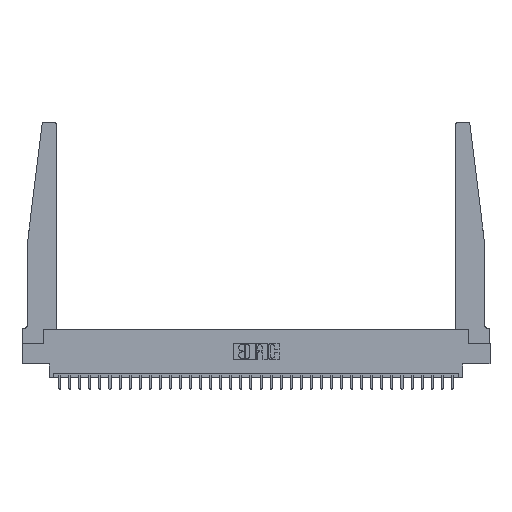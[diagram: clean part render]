
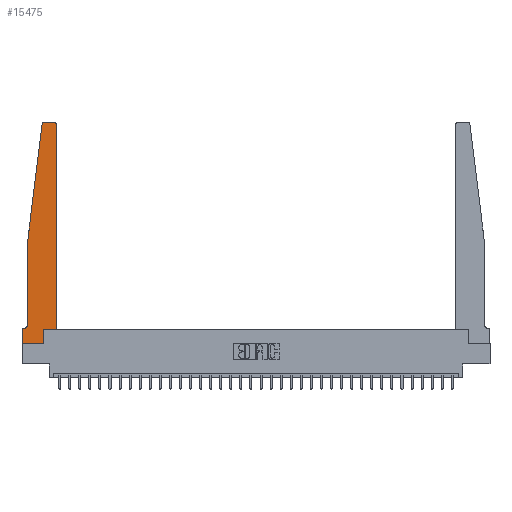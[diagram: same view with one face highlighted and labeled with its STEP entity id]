
A CAD part, top view. The second image highlights one B-rep face of the part: STEP entity #15475.
In plain terms, the highlighted planar face has unit normal (0, 0, 1).
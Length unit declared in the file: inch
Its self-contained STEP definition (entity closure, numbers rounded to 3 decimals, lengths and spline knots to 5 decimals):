
#81 = CARTESIAN_POINT ( 'NONE',  ( 0.395, 2.75, 0.37 ) ) ;
#188 = EDGE_CURVE ( 'NONE', #4004, #19025, #22978, .T. ) ;
#197 = ORIENTED_EDGE ( 'NONE', *, *, #20893, .T. ) ;
#679 = DIRECTION ( 'NONE',  ( 0., -1., 0. ) ) ;
#1126 = CARTESIAN_POINT ( 'NONE',  ( 0.425, 0.18, 0.37 ) ) ;
#2645 = CARTESIAN_POINT ( 'NONE',  ( 0.395, 2.72, 0.37 ) ) ;
#3099 = CARTESIAN_POINT ( 'NONE',  ( 0.065, 1.25, 0.37 ) ) ;
#3260 = CARTESIAN_POINT ( 'NONE',  ( 0.065, 1.25, 0.37 ) ) ;
#3842 = ORIENTED_EDGE ( 'NONE', *, *, #188, .T. ) ;
#3974 = DIRECTION ( 'NONE',  ( 1., 0., 0. ) ) ;
#4004 = VERTEX_POINT ( 'NONE', #18181 ) ;
#4383 = VERTEX_POINT ( 'NONE', #7712 ) ;
#4920 = VECTOR ( 'NONE', #15862, 39.37008 ) ;
#5093 = CARTESIAN_POINT ( 'NONE',  ( 0., 0., 0.37 ) ) ;
#5381 = ORIENTED_EDGE ( 'NONE', *, *, #17141, .T. ) ;
#5448 = VECTOR ( 'NONE', #679, 39.37008 ) ;
#6052 = EDGE_CURVE ( 'NONE', #19632, #29358, #28255, .T. ) ;
#6224 = EDGE_CURVE ( 'NONE', #10576, #30349, #29089, .T. ) ;
#6478 = VECTOR ( 'NONE', #3974, 39.37008 ) ;
#6811 = VERTEX_POINT ( 'NONE', #24458 ) ;
#6896 = CARTESIAN_POINT ( 'NONE',  ( 0.27653, 2.75, 0.37 ) ) ;
#7682 = DIRECTION ( 'NONE',  ( 1., 0., 0. ) ) ;
#7712 = CARTESIAN_POINT ( 'NONE',  ( 0.065, 1.25, 0.37 ) ) ;
#8177 = CARTESIAN_POINT ( 'NONE',  ( 0.2605, 0.18, 0.37 ) ) ;
#8314 = CARTESIAN_POINT ( 'NONE',  ( 0.25, 2.75, 0.37 ) ) ;
#8515 = DIRECTION ( 'NONE',  ( 0., -1., 0. ) ) ;
#9264 = CARTESIAN_POINT ( 'NONE',  ( 0., 0., 0.37 ) ) ;
#9479 = ORIENTED_EDGE ( 'NONE', *, *, #21279, .T. ) ;
#9689 = DIRECTION ( 'NONE',  ( 0., 0., 1. ) ) ;
#9752 = ORIENTED_EDGE ( 'NONE', *, *, #24899, .T. ) ;
#9802 = VECTOR ( 'NONE', #8515, 39.37008 ) ;
#10396 = ORIENTED_EDGE ( 'NONE', *, *, #6224, .T. ) ;
#10576 = VERTEX_POINT ( 'NONE', #6896 ) ;
#10902 = EDGE_CURVE ( 'NONE', #19761, #19632, #23251, .T. ) ;
#11032 = ORIENTED_EDGE ( 'NONE', *, *, #10902, .T. ) ;
#11674 = ORIENTED_EDGE ( 'NONE', *, *, #31141, .T. ) ;
#11796 = VECTOR ( 'NONE', #20056, 39.37008 ) ;
#12055 = CARTESIAN_POINT ( 'NONE',  ( 0.425, 0.18, 0.37 ) ) ;
#12337 = EDGE_CURVE ( 'NONE', #4383, #18650, #25102, .T. ) ;
#12482 = FACE_OUTER_BOUND ( 'NONE', #17894, .T. ) ;
#12603 = VECTOR ( 'NONE', #29712, 39.37008 ) ;
#12979 = CARTESIAN_POINT ( 'NONE',  ( 0.065, 0.1875, 0.37 ) ) ;
#14543 = LINE ( 'NONE', #5093, #21411 ) ;
#14899 = PLANE ( 'NONE',  #20337 ) ;
#15475 = ADVANCED_FACE ( 'NONE', ( #12482 ), #14899, .T. ) ;
#15824 = AXIS2_PLACEMENT_3D ( 'NONE', #2645, #9689, #31714 ) ;
#15862 = DIRECTION ( 'NONE',  ( 0., 1., 0. ) ) ;
#16350 = ORIENTED_EDGE ( 'NONE', *, *, #20463, .T. ) ;
#16833 = VECTOR ( 'NONE', #25554, 39.37008 ) ;
#17141 = EDGE_CURVE ( 'NONE', #29358, #25570, #25386, .T. ) ;
#17362 = CIRCLE ( 'NONE', #15824, 0.03 ) ;
#17663 = CARTESIAN_POINT ( 'NONE',  ( 0.2605, 0.18, 0.37 ) ) ;
#17666 = CARTESIAN_POINT ( 'NONE',  ( 0., 0., 0.37 ) ) ;
#17828 = CARTESIAN_POINT ( 'NONE',  ( 0.2605, 0., 0.37 ) ) ;
#17894 = EDGE_LOOP ( 'NONE', ( #9752, #10396, #197, #23150, #28321, #11674, #3842, #16350, #11032, #21083, #5381, #9479 ) ) ;
#18181 = CARTESIAN_POINT ( 'NONE',  ( 0., 0.1875, 0.37 ) ) ;
#18323 = DIRECTION ( 'NONE',  ( -0.122, -0.992, 0. ) ) ;
#18650 = VERTEX_POINT ( 'NONE', #29242 ) ;
#19025 = VERTEX_POINT ( 'NONE', #9264 ) ;
#19557 = CARTESIAN_POINT ( 'NONE',  ( 0., 0.1875, 0.37 ) ) ;
#19632 = VERTEX_POINT ( 'NONE', #17663 ) ;
#19761 = VERTEX_POINT ( 'NONE', #17828 ) ;
#19867 = LINE ( 'NONE', #8314, #12603 ) ;
#20056 = DIRECTION ( 'NONE',  ( -1., 0., 0. ) ) ;
#20337 = AXIS2_PLACEMENT_3D ( 'NONE', #19557, #29387, #7682 ) ;
#20463 = EDGE_CURVE ( 'NONE', #19025, #19761, #14543, .T. ) ;
#20893 = EDGE_CURVE ( 'NONE', #30349, #4383, #25420, .T. ) ;
#21083 = ORIENTED_EDGE ( 'NONE', *, *, #6052, .T. ) ;
#21279 = EDGE_CURVE ( 'NONE', #25570, #23945, #17362, .T. ) ;
#21411 = VECTOR ( 'NONE', #21940, 39.37008 ) ;
#21899 = CIRCLE ( 'NONE', #26031, 0.05 ) ;
#21940 = DIRECTION ( 'NONE',  ( 1., 0., 0. ) ) ;
#22890 = AXIS2_PLACEMENT_3D ( 'NONE', #23866, #29194, #26937 ) ;
#22978 = LINE ( 'NONE', #17666, #9802 ) ;
#23150 = ORIENTED_EDGE ( 'NONE', *, *, #12337, .T. ) ;
#23225 = DIRECTION ( 'NONE',  ( -1., 0., 0. ) ) ;
#23251 = LINE ( 'NONE', #8177, #4920 ) ;
#23556 = CARTESIAN_POINT ( 'NONE',  ( 0.015, 0.2375, 0.37 ) ) ;
#23717 = CARTESIAN_POINT ( 'NONE',  ( 0.425, 0.18, 0.37 ) ) ;
#23866 = CARTESIAN_POINT ( 'NONE',  ( 0.27653, 2.72, 0.37 ) ) ;
#23945 = VERTEX_POINT ( 'NONE', #81 ) ;
#24458 = CARTESIAN_POINT ( 'NONE',  ( 0.015, 0.1875, 0.37 ) ) ;
#24899 = EDGE_CURVE ( 'NONE', #23945, #10576, #19867, .T. ) ;
#25102 = LINE ( 'NONE', #3099, #5448 ) ;
#25386 = LINE ( 'NONE', #1126, #16833 ) ;
#25403 = EDGE_CURVE ( 'NONE', #18650, #6811, #21899, .T. ) ;
#25420 = LINE ( 'NONE', #3260, #26615 ) ;
#25554 = DIRECTION ( 'NONE',  ( 0., 1., 0. ) ) ;
#25570 = VERTEX_POINT ( 'NONE', #29027 ) ;
#25608 = CARTESIAN_POINT ( 'NONE',  ( 0.24675, 2.72367, 0.37 ) ) ;
#26031 = AXIS2_PLACEMENT_3D ( 'NONE', #23556, #27929, #23225 ) ;
#26615 = VECTOR ( 'NONE', #18323, 39.37008 ) ;
#26937 = DIRECTION ( 'NONE',  ( 1., 0., 0. ) ) ;
#27929 = DIRECTION ( 'NONE',  ( 0., 0., -1. ) ) ;
#28255 = LINE ( 'NONE', #23717, #6478 ) ;
#28321 = ORIENTED_EDGE ( 'NONE', *, *, #25403, .T. ) ;
#29027 = CARTESIAN_POINT ( 'NONE',  ( 0.425, 2.72, 0.37 ) ) ;
#29089 = CIRCLE ( 'NONE', #22890, 0.03 ) ;
#29194 = DIRECTION ( 'NONE',  ( 0., 0., 1. ) ) ;
#29242 = CARTESIAN_POINT ( 'NONE',  ( 0.065, 0.2375, 0.37 ) ) ;
#29358 = VERTEX_POINT ( 'NONE', #12055 ) ;
#29387 = DIRECTION ( 'NONE',  ( 0., 0., 1. ) ) ;
#29712 = DIRECTION ( 'NONE',  ( -1., 0., 0. ) ) ;
#30201 = LINE ( 'NONE', #12979, #11796 ) ;
#30349 = VERTEX_POINT ( 'NONE', #25608 ) ;
#31141 = EDGE_CURVE ( 'NONE', #6811, #4004, #30201, .T. ) ;
#31714 = DIRECTION ( 'NONE',  ( 1., 0., 0. ) ) ;
